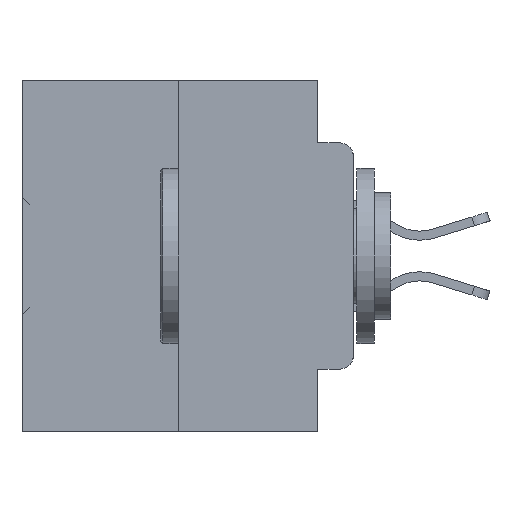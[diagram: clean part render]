
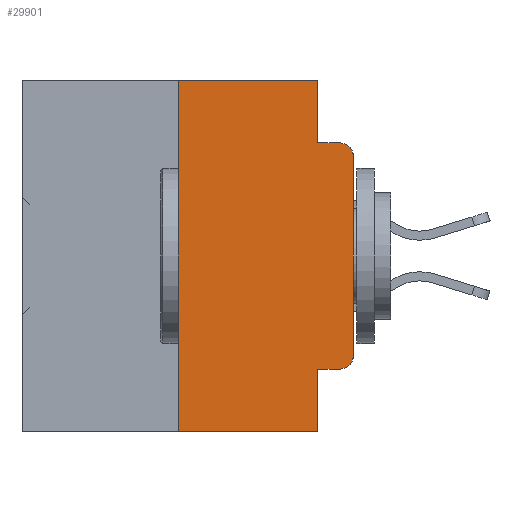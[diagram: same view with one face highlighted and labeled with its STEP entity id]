
A CAD part, left-side view. The second image highlights one B-rep face of the part: STEP entity #29901.
In plain terms, the highlighted planar face has unit normal (-1, 0, 0).
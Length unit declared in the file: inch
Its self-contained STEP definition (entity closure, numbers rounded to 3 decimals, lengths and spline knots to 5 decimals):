
#842 = DIRECTION ( 'NONE',  ( 0., -1., 0. ) ) ;
#1110 = DIRECTION ( 'NONE',  ( 0., 0., 1. ) ) ;
#1259 = LINE ( 'NONE', #16252, #24930 ) ;
#1583 = VECTOR ( 'NONE', #21327, 39.37008 ) ;
#1974 = EDGE_CURVE ( 'NONE', #7820, #35653, #1259, .T. ) ;
#2350 = ORIENTED_EDGE ( 'NONE', *, *, #27597, .T. ) ;
#2888 = CARTESIAN_POINT ( 'NONE',  ( 0., 0.473, 0. ) ) ;
#3218 = ORIENTED_EDGE ( 'NONE', *, *, #39839, .T. ) ;
#3815 = VECTOR ( 'NONE', #18547, 39.37008 ) ;
#3894 = CARTESIAN_POINT ( 'NONE',  ( 0., 0.051, -0.4115 ) ) ;
#4524 = VERTEX_POINT ( 'NONE', #36602 ) ;
#4584 = CARTESIAN_POINT ( 'NONE',  ( 0., 0.02, -0.1085 ) ) ;
#4613 = VECTOR ( 'NONE', #9076, 39.37008 ) ;
#5100 = ORIENTED_EDGE ( 'NONE', *, *, #13151, .T. ) ;
#5381 = CARTESIAN_POINT ( 'NONE',  ( 0., 0.25, -0.5 ) ) ;
#5466 = AXIS2_PLACEMENT_3D ( 'NONE', #14150, #23397, #23241 ) ;
#5573 = DIRECTION ( 'NONE',  ( 0., -1., 0. ) ) ;
#5646 = CARTESIAN_POINT ( 'NONE',  ( 0., 0., -0.3915 ) ) ;
#5841 = LINE ( 'NONE', #10255, #33480 ) ;
#5988 = LINE ( 'NONE', #33640, #4613 ) ;
#6637 = LINE ( 'NONE', #7570, #36715 ) ;
#7570 = CARTESIAN_POINT ( 'NONE',  ( 0., 0.473, -0.5 ) ) ;
#7820 = VERTEX_POINT ( 'NONE', #8678 ) ;
#7842 = EDGE_CURVE ( 'NONE', #22022, #10737, #5988, .T. ) ;
#8678 = CARTESIAN_POINT ( 'NONE',  ( 0., 0.051, 0. ) ) ;
#9076 = DIRECTION ( 'NONE',  ( 0., 0., 1. ) ) ;
#9565 = LINE ( 'NONE', #36615, #3815 ) ;
#9641 = VERTEX_POINT ( 'NONE', #36887 ) ;
#9699 = EDGE_LOOP ( 'NONE', ( #22902, #12715, #33534, #37622, #36750, #11040, #2350, #26610, #3218, #5100 ) ) ;
#10255 = CARTESIAN_POINT ( 'NONE',  ( 0., 0.25, 0. ) ) ;
#10737 = VERTEX_POINT ( 'NONE', #29379 ) ;
#11040 = ORIENTED_EDGE ( 'NONE', *, *, #31392, .F. ) ;
#12108 = DIRECTION ( 'NONE',  ( 0., -1., 0. ) ) ;
#12239 = CARTESIAN_POINT ( 'NONE',  ( 0., 0.473, 0. ) ) ;
#12715 = ORIENTED_EDGE ( 'NONE', *, *, #38278, .T. ) ;
#13151 = EDGE_CURVE ( 'NONE', #9641, #22022, #17799, .T. ) ;
#14150 = CARTESIAN_POINT ( 'NONE',  ( 0., 0.02, -0.3915 ) ) ;
#15074 = CARTESIAN_POINT ( 'NONE',  ( 0., 0.051, -0.0885 ) ) ;
#15236 = VERTEX_POINT ( 'NONE', #21954 ) ;
#16019 = VERTEX_POINT ( 'NONE', #29544 ) ;
#16252 = CARTESIAN_POINT ( 'NONE',  ( 0., 0.051, 0. ) ) ;
#17799 = CIRCLE ( 'NONE', #5466, 0.02 ) ;
#18352 = CARTESIAN_POINT ( 'NONE',  ( 0., 0.051, -0.0885 ) ) ;
#18547 = DIRECTION ( 'NONE',  ( 0., 0., -1. ) ) ;
#18676 = LINE ( 'NONE', #2888, #29868 ) ;
#19936 = AXIS2_PLACEMENT_3D ( 'NONE', #4584, #39074, #38664 ) ;
#20456 = VERTEX_POINT ( 'NONE', #3894 ) ;
#21327 = DIRECTION ( 'NONE',  ( 0., -1., 0. ) ) ;
#21633 = DIRECTION ( 'NONE',  ( 1., 0., 0. ) ) ;
#21886 = LINE ( 'NONE', #30412, #1583 ) ;
#21954 = CARTESIAN_POINT ( 'NONE',  ( 0., 0.02, -0.0885 ) ) ;
#22022 = VERTEX_POINT ( 'NONE', #5646 ) ;
#22454 = FACE_OUTER_BOUND ( 'NONE', #9699, .T. ) ;
#22902 = ORIENTED_EDGE ( 'NONE', *, *, #7842, .T. ) ;
#23241 = DIRECTION ( 'NONE',  ( 0., 0., -1. ) ) ;
#23397 = DIRECTION ( 'NONE',  ( -1., 0., 0. ) ) ;
#23703 = VECTOR ( 'NONE', #12108, 39.37008 ) ;
#24339 = DIRECTION ( 'NONE',  ( 0., 0., -1. ) ) ;
#24930 = VECTOR ( 'NONE', #31882, 39.37008 ) ;
#25047 = EDGE_CURVE ( 'NONE', #20456, #16019, #9565, .T. ) ;
#25901 = EDGE_CURVE ( 'NONE', #35653, #15236, #33887, .T. ) ;
#26610 = ORIENTED_EDGE ( 'NONE', *, *, #25047, .F. ) ;
#27597 = EDGE_CURVE ( 'NONE', #37447, #16019, #6637, .T. ) ;
#28293 = AXIS2_PLACEMENT_3D ( 'NONE', #12239, #21633, #24339 ) ;
#29379 = CARTESIAN_POINT ( 'NONE',  ( 0., 0., -0.1085 ) ) ;
#29544 = CARTESIAN_POINT ( 'NONE',  ( 0., 0.051, -0.5 ) ) ;
#29868 = VECTOR ( 'NONE', #5573, 39.37008 ) ;
#29901 = ADVANCED_FACE ( 'NONE', ( #22454 ), #37203, .F. ) ;
#30412 = CARTESIAN_POINT ( 'NONE',  ( 0., 0.051, -0.4115 ) ) ;
#31392 = EDGE_CURVE ( 'NONE', #37447, #4524, #5841, .T. ) ;
#31488 = CIRCLE ( 'NONE', #19936, 0.02 ) ;
#31882 = DIRECTION ( 'NONE',  ( 0., 0., -1. ) ) ;
#33480 = VECTOR ( 'NONE', #1110, 39.37008 ) ;
#33534 = ORIENTED_EDGE ( 'NONE', *, *, #25901, .F. ) ;
#33640 = CARTESIAN_POINT ( 'NONE',  ( 0., 0., 0. ) ) ;
#33887 = LINE ( 'NONE', #18352, #23703 ) ;
#34383 = EDGE_CURVE ( 'NONE', #4524, #7820, #18676, .T. ) ;
#35653 = VERTEX_POINT ( 'NONE', #15074 ) ;
#36602 = CARTESIAN_POINT ( 'NONE',  ( 0., 0.25, 0. ) ) ;
#36615 = CARTESIAN_POINT ( 'NONE',  ( 0., 0.051, 0. ) ) ;
#36715 = VECTOR ( 'NONE', #842, 39.37008 ) ;
#36750 = ORIENTED_EDGE ( 'NONE', *, *, #34383, .F. ) ;
#36887 = CARTESIAN_POINT ( 'NONE',  ( 0., 0.02, -0.4115 ) ) ;
#37203 = PLANE ( 'NONE',  #28293 ) ;
#37447 = VERTEX_POINT ( 'NONE', #5381 ) ;
#37622 = ORIENTED_EDGE ( 'NONE', *, *, #1974, .F. ) ;
#38278 = EDGE_CURVE ( 'NONE', #10737, #15236, #31488, .T. ) ;
#38664 = DIRECTION ( 'NONE',  ( 0., 0., -1. ) ) ;
#39074 = DIRECTION ( 'NONE',  ( -1., 0., 0. ) ) ;
#39839 = EDGE_CURVE ( 'NONE', #20456, #9641, #21886, .T. ) ;
